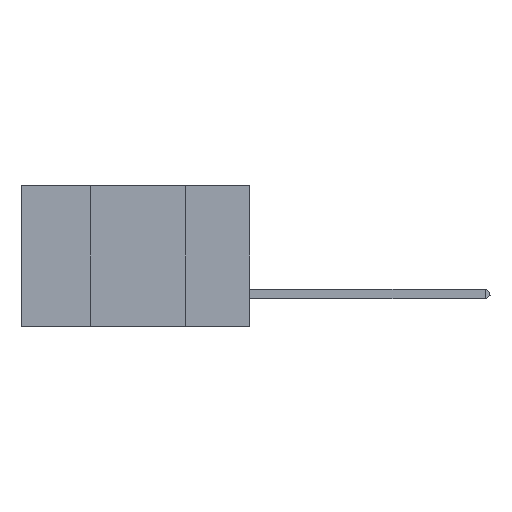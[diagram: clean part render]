
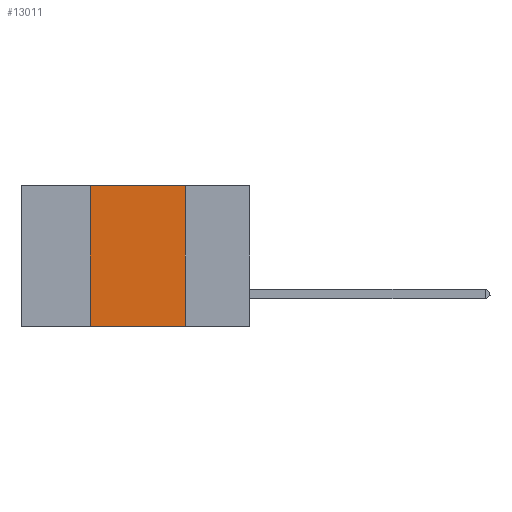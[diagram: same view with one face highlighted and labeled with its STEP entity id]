
A CAD part, left-side view. The second image highlights one B-rep face of the part: STEP entity #13011.
In plain terms, the highlighted planar face has unit normal (-1, 0, 0).
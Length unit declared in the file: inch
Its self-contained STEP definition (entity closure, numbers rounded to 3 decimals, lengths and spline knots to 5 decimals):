
#719 = CARTESIAN_POINT ( 'NONE',  ( 0., 0.17, 0. ) ) ;
#730 = VECTOR ( 'NONE', #23255, 39.37008 ) ;
#1127 = CARTESIAN_POINT ( 'NONE',  ( 0., 0.6, 0. ) ) ;
#1903 = CARTESIAN_POINT ( 'NONE',  ( 0., 0.42, -0.37 ) ) ;
#2953 = DIRECTION ( 'NONE',  ( 0., 0., -1. ) ) ;
#3475 = LINE ( 'NONE', #1127, #22803 ) ;
#3478 = VECTOR ( 'NONE', #13647, 39.37008 ) ;
#4413 = ORIENTED_EDGE ( 'NONE', *, *, #14021, .F. ) ;
#4972 = CARTESIAN_POINT ( 'NONE',  ( 0., 0.6, -0.37 ) ) ;
#5562 = VERTEX_POINT ( 'NONE', #9165 ) ;
#5742 = LINE ( 'NONE', #719, #730 ) ;
#5968 = EDGE_CURVE ( 'NONE', #21653, #11386, #7879, .T. ) ;
#6865 = ORIENTED_EDGE ( 'NONE', *, *, #23205, .T. ) ;
#7052 = DIRECTION ( 'NONE',  ( 0., -1., 0. ) ) ;
#7856 = CARTESIAN_POINT ( 'NONE',  ( 0., 0.42, 0. ) ) ;
#7879 = LINE ( 'NONE', #7856, #3478 ) ;
#8789 = DIRECTION ( 'NONE',  ( 0., -1., 0. ) ) ;
#9165 = CARTESIAN_POINT ( 'NONE',  ( 0., 0.17, -0.37 ) ) ;
#9594 = VECTOR ( 'NONE', #8789, 39.37008 ) ;
#11081 = PLANE ( 'NONE',  #15049 ) ;
#11386 = VERTEX_POINT ( 'NONE', #20377 ) ;
#13011 = ADVANCED_FACE ( 'NONE', ( #17872 ), #11081, .F. ) ;
#13447 = CARTESIAN_POINT ( 'NONE',  ( 0., 0.6, 0. ) ) ;
#13647 = DIRECTION ( 'NONE',  ( 0., 0., 1. ) ) ;
#14021 = EDGE_CURVE ( 'NONE', #11386, #22181, #3475, .T. ) ;
#14555 = LINE ( 'NONE', #4972, #9594 ) ;
#15049 = AXIS2_PLACEMENT_3D ( 'NONE', #13447, #15298, #2953 ) ;
#15298 = DIRECTION ( 'NONE',  ( 1., 0., 0. ) ) ;
#15344 = ORIENTED_EDGE ( 'NONE', *, *, #19597, .F. ) ;
#16495 = EDGE_LOOP ( 'NONE', ( #15344, #4413, #18536, #6865 ) ) ;
#17872 = FACE_OUTER_BOUND ( 'NONE', #16495, .T. ) ;
#18536 = ORIENTED_EDGE ( 'NONE', *, *, #5968, .F. ) ;
#18616 = CARTESIAN_POINT ( 'NONE',  ( 0., 0.17, 0. ) ) ;
#19597 = EDGE_CURVE ( 'NONE', #22181, #5562, #5742, .T. ) ;
#20377 = CARTESIAN_POINT ( 'NONE',  ( 0., 0.42, 0. ) ) ;
#21653 = VERTEX_POINT ( 'NONE', #1903 ) ;
#22181 = VERTEX_POINT ( 'NONE', #18616 ) ;
#22803 = VECTOR ( 'NONE', #7052, 39.37008 ) ;
#23205 = EDGE_CURVE ( 'NONE', #21653, #5562, #14555, .T. ) ;
#23255 = DIRECTION ( 'NONE',  ( 0., 0., -1. ) ) ;
